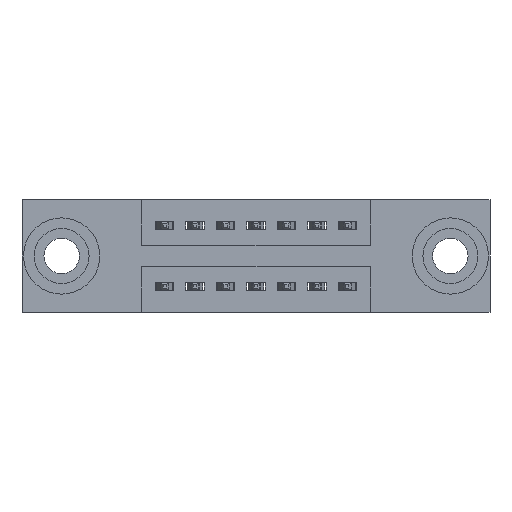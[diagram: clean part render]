
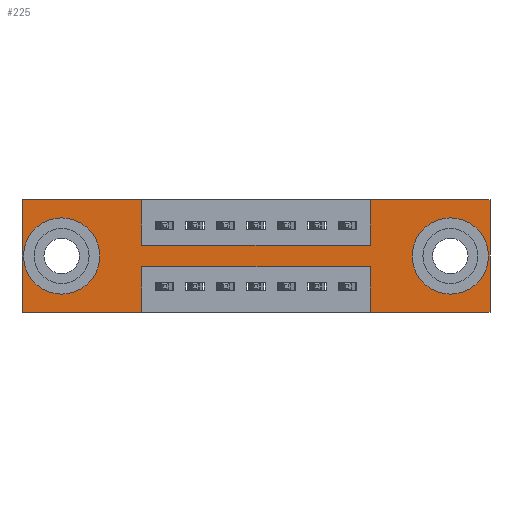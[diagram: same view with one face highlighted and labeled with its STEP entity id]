
A CAD part, front view. The second image highlights one B-rep face of the part: STEP entity #225.
In plain terms, the highlighted planar face has unit normal (0, -1, 0).
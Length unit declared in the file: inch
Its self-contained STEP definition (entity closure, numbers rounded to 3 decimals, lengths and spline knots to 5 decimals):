
#13 = FACE_BOUND ( 'NONE', #2120, .T. ) ;
#18 = DIRECTION ( 'NONE',  ( 0., 0., -1. ) ) ;
#107 = CARTESIAN_POINT ( 'NONE',  ( 0.13, 0., -0.263 ) ) ;
#179 = VECTOR ( 'NONE', #7263, 39.37008 ) ;
#198 = CIRCLE ( 'NONE', #5250, 0.078 ) ;
#225 = ADVANCED_FACE ( 'NONE', ( #2731, #13, #7245 ), #1965, .T. ) ;
#291 = ORIENTED_EDGE ( 'NONE', *, *, #8839, .F. ) ;
#323 = VERTEX_POINT ( 'NONE', #3693 ) ;
#591 = VERTEX_POINT ( 'NONE', #6399 ) ;
#627 = VECTOR ( 'NONE', #9979, 39.37008 ) ;
#723 = DIRECTION ( 'NONE',  ( 0., 0., 1. ) ) ;
#783 = EDGE_CURVE ( 'NONE', #2665, #5066, #8672, .T. ) ;
#811 = ORIENTED_EDGE ( 'NONE', *, *, #4228, .F. ) ;
#829 = VERTEX_POINT ( 'NONE', #1157 ) ;
#857 = CARTESIAN_POINT ( 'NONE',  ( 1.405, 0., -0.185 ) ) ;
#1059 = CARTESIAN_POINT ( 'NONE',  ( 0., 0., -0.37 ) ) ;
#1157 = CARTESIAN_POINT ( 'NONE',  ( 1.535, 0., -0.37 ) ) ;
#1253 = CARTESIAN_POINT ( 'NONE',  ( 0.3925, 0., -0.37 ) ) ;
#1535 = CARTESIAN_POINT ( 'NONE',  ( 0., 0., -0.37 ) ) ;
#1589 = ORIENTED_EDGE ( 'NONE', *, *, #8098, .T. ) ;
#1691 = EDGE_LOOP ( 'NONE', ( #4745, #2188, #4060, #5939, #291, #9845, #811, #5339, #9515, #2771, #7887, #6910 ) ) ;
#1721 = LINE ( 'NONE', #1535, #4721 ) ;
#1788 = CARTESIAN_POINT ( 'NONE',  ( 0.3925, 0., -0.37 ) ) ;
#1900 = VERTEX_POINT ( 'NONE', #1788 ) ;
#1901 = EDGE_CURVE ( 'NONE', #2735, #8899, #10752, .T. ) ;
#1935 = DIRECTION ( 'NONE',  ( 0., 0., -1. ) ) ;
#1952 = VECTOR ( 'NONE', #3777, 39.37008 ) ;
#1965 = PLANE ( 'NONE',  #7152 ) ;
#2120 = EDGE_LOOP ( 'NONE', ( #4790, #2564 ) ) ;
#2188 = ORIENTED_EDGE ( 'NONE', *, *, #8724, .F. ) ;
#2199 = LINE ( 'NONE', #6774, #8010 ) ;
#2304 = EDGE_CURVE ( 'NONE', #2506, #8617, #2308, .T. ) ;
#2308 = LINE ( 'NONE', #4183, #627 ) ;
#2371 = DIRECTION ( 'NONE',  ( -1., 0., 0. ) ) ;
#2506 = VERTEX_POINT ( 'NONE', #7540 ) ;
#2513 = CARTESIAN_POINT ( 'NONE',  ( 0., 0., 0. ) ) ;
#2564 = ORIENTED_EDGE ( 'NONE', *, *, #4679, .T. ) ;
#2665 = VERTEX_POINT ( 'NONE', #4010 ) ;
#2669 = DIRECTION ( 'NONE',  ( 0., 0., 1. ) ) ;
#2681 = VECTOR ( 'NONE', #8313, 39.37008 ) ;
#2731 = FACE_BOUND ( 'NONE', #7948, .T. ) ;
#2735 = VERTEX_POINT ( 'NONE', #9693 ) ;
#2756 = DIRECTION ( 'NONE',  ( 0., 1., 0. ) ) ;
#2771 = ORIENTED_EDGE ( 'NONE', *, *, #9921, .F. ) ;
#2820 = CARTESIAN_POINT ( 'NONE',  ( 1.535, 0., 0. ) ) ;
#3441 = DIRECTION ( 'NONE',  ( 0., 0., -1. ) ) ;
#3479 = EDGE_CURVE ( 'NONE', #323, #1900, #10457, .T. ) ;
#3546 = VECTOR ( 'NONE', #3441, 39.37008 ) ;
#3566 = CIRCLE ( 'NONE', #7175, 0.078 ) ;
#3604 = CARTESIAN_POINT ( 'NONE',  ( 1.405, 0., -0.263 ) ) ;
#3658 = VERTEX_POINT ( 'NONE', #5593 ) ;
#3693 = CARTESIAN_POINT ( 'NONE',  ( 0.3925, 0., -0.22 ) ) ;
#3707 = EDGE_CURVE ( 'NONE', #3658, #9312, #2199, .T. ) ;
#3777 = DIRECTION ( 'NONE',  ( 1., 0., 0. ) ) ;
#4010 = CARTESIAN_POINT ( 'NONE',  ( 1.1425, 0., 0. ) ) ;
#4060 = ORIENTED_EDGE ( 'NONE', *, *, #5843, .F. ) ;
#4183 = CARTESIAN_POINT ( 'NONE',  ( 0.3925, 0., -0.15 ) ) ;
#4214 = EDGE_CURVE ( 'NONE', #6648, #2506, #8512, .T. ) ;
#4228 = EDGE_CURVE ( 'NONE', #8617, #2665, #6406, .T. ) ;
#4337 = VECTOR ( 'NONE', #10518, 39.37008 ) ;
#4570 = CARTESIAN_POINT ( 'NONE',  ( 0., 0., -0.37 ) ) ;
#4619 = LINE ( 'NONE', #10601, #179 ) ;
#4679 = EDGE_CURVE ( 'NONE', #8899, #2735, #7858, .T. ) ;
#4721 = VECTOR ( 'NONE', #2371, 39.37008 ) ;
#4745 = ORIENTED_EDGE ( 'NONE', *, *, #3479, .F. ) ;
#4781 = ORIENTED_EDGE ( 'NONE', *, *, #5027, .T. ) ;
#4790 = ORIENTED_EDGE ( 'NONE', *, *, #1901, .T. ) ;
#4794 = CARTESIAN_POINT ( 'NONE',  ( 0.13, 0., -0.185 ) ) ;
#4808 = CARTESIAN_POINT ( 'NONE',  ( 1.1425, 0., -0.22 ) ) ;
#5027 = EDGE_CURVE ( 'NONE', #591, #8216, #198, .T. ) ;
#5066 = VERTEX_POINT ( 'NONE', #2820 ) ;
#5097 = CARTESIAN_POINT ( 'NONE',  ( 0.13, 0., -0.185 ) ) ;
#5224 = VERTEX_POINT ( 'NONE', #4808 ) ;
#5231 = LINE ( 'NONE', #6645, #9468 ) ;
#5250 = AXIS2_PLACEMENT_3D ( 'NONE', #6277, #2756, #1935 ) ;
#5339 = ORIENTED_EDGE ( 'NONE', *, *, #2304, .F. ) ;
#5574 = CARTESIAN_POINT ( 'NONE',  ( 1.1425, 0., -0.15 ) ) ;
#5593 = CARTESIAN_POINT ( 'NONE',  ( 0., 0., -0.37 ) ) ;
#5785 = CARTESIAN_POINT ( 'NONE',  ( 1.1425, 0., 0. ) ) ;
#5843 = EDGE_CURVE ( 'NONE', #9271, #5224, #4619, .T. ) ;
#5880 = VECTOR ( 'NONE', #8438, 39.37008 ) ;
#5909 = DIRECTION ( 'NONE',  ( 0., 1., 0. ) ) ;
#5937 = CARTESIAN_POINT ( 'NONE',  ( 1.535, 0., 0. ) ) ;
#5939 = ORIENTED_EDGE ( 'NONE', *, *, #10581, .F. ) ;
#6277 = CARTESIAN_POINT ( 'NONE',  ( 1.405, 0., -0.185 ) ) ;
#6396 = EDGE_CURVE ( 'NONE', #1900, #3658, #8600, .T. ) ;
#6399 = CARTESIAN_POINT ( 'NONE',  ( 1.405, 0., -0.107 ) ) ;
#6406 = LINE ( 'NONE', #5785, #10231 ) ;
#6531 = CARTESIAN_POINT ( 'NONE',  ( 1.1425, 0., -0.37 ) ) ;
#6618 = AXIS2_PLACEMENT_3D ( 'NONE', #4794, #9923, #723 ) ;
#6645 = CARTESIAN_POINT ( 'NONE',  ( 0.3925, 0., -0.22 ) ) ;
#6648 = VERTEX_POINT ( 'NONE', #10626 ) ;
#6774 = CARTESIAN_POINT ( 'NONE',  ( 0., 0., 0. ) ) ;
#6817 = DIRECTION ( 'NONE',  ( 0., 1., 0. ) ) ;
#6910 = ORIENTED_EDGE ( 'NONE', *, *, #6396, .F. ) ;
#7152 = AXIS2_PLACEMENT_3D ( 'NONE', #1059, #9434, #9511 ) ;
#7175 = AXIS2_PLACEMENT_3D ( 'NONE', #857, #5909, #18 ) ;
#7209 = DIRECTION ( 'NONE',  ( 0., 0., -1. ) ) ;
#7245 = FACE_OUTER_BOUND ( 'NONE', #1691, .T. ) ;
#7263 = DIRECTION ( 'NONE',  ( 0., 0., 1. ) ) ;
#7410 = CARTESIAN_POINT ( 'NONE',  ( 0., 0., 0. ) ) ;
#7540 = CARTESIAN_POINT ( 'NONE',  ( 0.3925, 0., -0.15 ) ) ;
#7679 = DIRECTION ( 'NONE',  ( 0., 0., 1. ) ) ;
#7858 = CIRCLE ( 'NONE', #6618, 0.078 ) ;
#7887 = ORIENTED_EDGE ( 'NONE', *, *, #3707, .F. ) ;
#7948 = EDGE_LOOP ( 'NONE', ( #4781, #1589 ) ) ;
#8010 = VECTOR ( 'NONE', #2669, 39.37008 ) ;
#8098 = EDGE_CURVE ( 'NONE', #8216, #591, #3566, .T. ) ;
#8216 = VERTEX_POINT ( 'NONE', #3604 ) ;
#8313 = DIRECTION ( 'NONE',  ( 0., 0., -1. ) ) ;
#8438 = DIRECTION ( 'NONE',  ( 1., 0., 0. ) ) ;
#8512 = LINE ( 'NONE', #10008, #2681 ) ;
#8600 = LINE ( 'NONE', #4570, #4337 ) ;
#8617 = VERTEX_POINT ( 'NONE', #5574 ) ;
#8672 = LINE ( 'NONE', #10634, #1952 ) ;
#8724 = EDGE_CURVE ( 'NONE', #5224, #323, #5231, .T. ) ;
#8839 = EDGE_CURVE ( 'NONE', #5066, #829, #10272, .T. ) ;
#8899 = VERTEX_POINT ( 'NONE', #107 ) ;
#8926 = LINE ( 'NONE', #2513, #5880 ) ;
#9191 = DIRECTION ( 'NONE',  ( -1., 0., 0. ) ) ;
#9271 = VERTEX_POINT ( 'NONE', #6531 ) ;
#9273 = AXIS2_PLACEMENT_3D ( 'NONE', #5097, #6817, #7679 ) ;
#9312 = VERTEX_POINT ( 'NONE', #7410 ) ;
#9434 = DIRECTION ( 'NONE',  ( 0., -1., 0. ) ) ;
#9468 = VECTOR ( 'NONE', #9191, 39.37008 ) ;
#9511 = DIRECTION ( 'NONE',  ( 0., 0., -1. ) ) ;
#9515 = ORIENTED_EDGE ( 'NONE', *, *, #4214, .F. ) ;
#9693 = CARTESIAN_POINT ( 'NONE',  ( 0.13, 0., -0.107 ) ) ;
#9845 = ORIENTED_EDGE ( 'NONE', *, *, #783, .F. ) ;
#9921 = EDGE_CURVE ( 'NONE', #9312, #6648, #8926, .T. ) ;
#9923 = DIRECTION ( 'NONE',  ( 0., 1., 0. ) ) ;
#9979 = DIRECTION ( 'NONE',  ( 1., 0., 0. ) ) ;
#10008 = CARTESIAN_POINT ( 'NONE',  ( 0.3925, 0., 0. ) ) ;
#10079 = DIRECTION ( 'NONE',  ( 0., 0., 1. ) ) ;
#10231 = VECTOR ( 'NONE', #10079, 39.37008 ) ;
#10272 = LINE ( 'NONE', #5937, #3546 ) ;
#10352 = VECTOR ( 'NONE', #7209, 39.37008 ) ;
#10457 = LINE ( 'NONE', #1253, #10352 ) ;
#10518 = DIRECTION ( 'NONE',  ( -1., 0., 0. ) ) ;
#10581 = EDGE_CURVE ( 'NONE', #829, #9271, #1721, .T. ) ;
#10601 = CARTESIAN_POINT ( 'NONE',  ( 1.1425, 0., -0.37 ) ) ;
#10626 = CARTESIAN_POINT ( 'NONE',  ( 0.3925, 0., 0. ) ) ;
#10634 = CARTESIAN_POINT ( 'NONE',  ( 0., 0., 0. ) ) ;
#10752 = CIRCLE ( 'NONE', #9273, 0.078 ) ;
